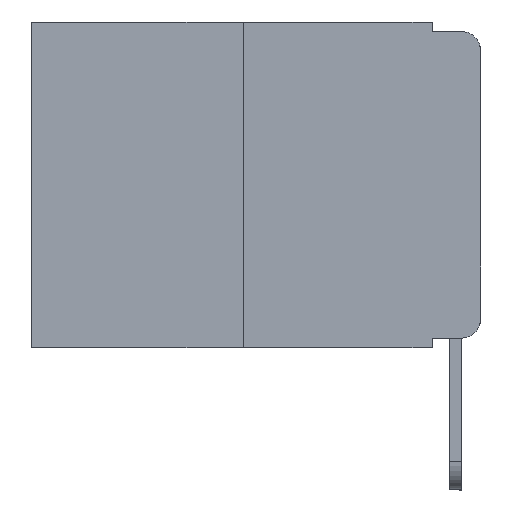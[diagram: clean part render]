
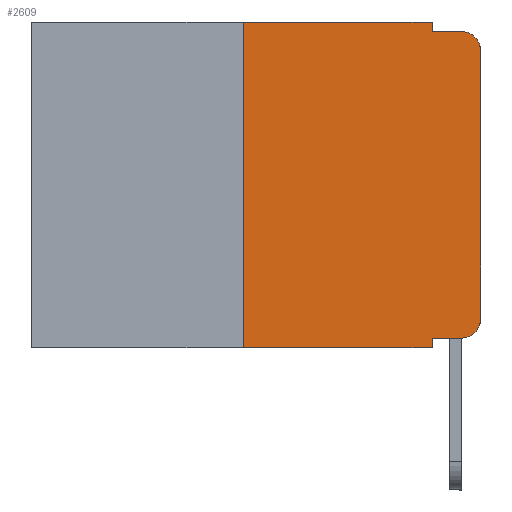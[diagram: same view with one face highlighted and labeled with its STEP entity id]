
A CAD part, left-side view. The second image highlights one B-rep face of the part: STEP entity #2609.
In plain terms, the highlighted planar face has unit normal (-1, 0, 0).
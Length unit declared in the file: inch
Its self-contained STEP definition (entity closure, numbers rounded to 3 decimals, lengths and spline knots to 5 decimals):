
#767 = DIRECTION ( 'NONE',  ( 0., 0., 1. ) ) ;
#901 = AXIS2_PLACEMENT_3D ( 'NONE', #13394, #9608, #2541 ) ;
#1169 = LINE ( 'NONE', #12186, #2252 ) ;
#1453 = VERTEX_POINT ( 'NONE', #3681 ) ;
#1480 = VECTOR ( 'NONE', #8180, 39.37008 ) ;
#2252 = VECTOR ( 'NONE', #17373, 39.37008 ) ;
#2254 = CARTESIAN_POINT ( 'NONE',  ( 0., 0.25, 0. ) ) ;
#2541 = DIRECTION ( 'NONE',  ( 0., 0., -1. ) ) ;
#2609 = ADVANCED_FACE ( 'NONE', ( #9965 ), #8633, .F. ) ;
#2636 = CARTESIAN_POINT ( 'NONE',  ( 0., 0.473, -0.343 ) ) ;
#3166 = EDGE_CURVE ( 'NONE', #3758, #8731, #11826, .T. ) ;
#3441 = EDGE_LOOP ( 'NONE', ( #13390, #12793, #8458, #8248, #9244, #13747, #9294, #8900, #12573, #4435 ) ) ;
#3514 = LINE ( 'NONE', #11663, #14878 ) ;
#3665 = EDGE_CURVE ( 'NONE', #16578, #8731, #12318, .T. ) ;
#3681 = CARTESIAN_POINT ( 'NONE',  ( 0., 0., -0.313 ) ) ;
#3758 = VERTEX_POINT ( 'NONE', #12150 ) ;
#3892 = CARTESIAN_POINT ( 'NONE',  ( 0., 0.051, -0.333 ) ) ;
#4093 = VERTEX_POINT ( 'NONE', #13657 ) ;
#4435 = ORIENTED_EDGE ( 'NONE', *, *, #17539, .T. ) ;
#4487 = DIRECTION ( 'NONE',  ( 0., -1., 0. ) ) ;
#4584 = VECTOR ( 'NONE', #4487, 39.37008 ) ;
#4622 = CARTESIAN_POINT ( 'NONE',  ( 0., 0., 0. ) ) ;
#4822 = CARTESIAN_POINT ( 'NONE',  ( 0., 0.02, -0.01 ) ) ;
#5192 = CARTESIAN_POINT ( 'NONE',  ( 0., 0.02, -0.03 ) ) ;
#5242 = VERTEX_POINT ( 'NONE', #5720 ) ;
#5525 = DIRECTION ( 'NONE',  ( 1., 0., 0. ) ) ;
#5674 = VERTEX_POINT ( 'NONE', #3892 ) ;
#5720 = CARTESIAN_POINT ( 'NONE',  ( 0., 0.02, -0.333 ) ) ;
#5815 = EDGE_CURVE ( 'NONE', #1453, #3758, #6295, .T. ) ;
#6295 = LINE ( 'NONE', #4622, #10656 ) ;
#7098 = LINE ( 'NONE', #8301, #13441 ) ;
#7421 = DIRECTION ( 'NONE',  ( 0., 0., 1. ) ) ;
#8180 = DIRECTION ( 'NONE',  ( 0., -1., 0. ) ) ;
#8186 = DIRECTION ( 'NONE',  ( 0., -1., 0. ) ) ;
#8248 = ORIENTED_EDGE ( 'NONE', *, *, #11457, .F. ) ;
#8301 = CARTESIAN_POINT ( 'NONE',  ( 0., 0.051, 0. ) ) ;
#8458 = ORIENTED_EDGE ( 'NONE', *, *, #3665, .F. ) ;
#8633 = PLANE ( 'NONE',  #9193 ) ;
#8731 = VERTEX_POINT ( 'NONE', #4822 ) ;
#8786 = DIRECTION ( 'NONE',  ( -1., 0., 0. ) ) ;
#8900 = ORIENTED_EDGE ( 'NONE', *, *, #15460, .F. ) ;
#8952 = AXIS2_PLACEMENT_3D ( 'NONE', #5192, #8786, #13424 ) ;
#8954 = VECTOR ( 'NONE', #767, 39.37008 ) ;
#8999 = CARTESIAN_POINT ( 'NONE',  ( 0., 0.25, 0. ) ) ;
#9193 = AXIS2_PLACEMENT_3D ( 'NONE', #14134, #5525, #16583 ) ;
#9244 = ORIENTED_EDGE ( 'NONE', *, *, #15799, .F. ) ;
#9294 = ORIENTED_EDGE ( 'NONE', *, *, #17681, .T. ) ;
#9521 = LINE ( 'NONE', #2636, #1480 ) ;
#9608 = DIRECTION ( 'NONE',  ( -1., 0., 0. ) ) ;
#9965 = FACE_OUTER_BOUND ( 'NONE', #3441, .T. ) ;
#10115 = VERTEX_POINT ( 'NONE', #16074 ) ;
#10433 = LINE ( 'NONE', #8999, #8954 ) ;
#10656 = VECTOR ( 'NONE', #7421, 39.37008 ) ;
#10741 = EDGE_CURVE ( 'NONE', #5674, #5242, #3514, .T. ) ;
#10966 = CARTESIAN_POINT ( 'NONE',  ( 0., 0.051, -0.01 ) ) ;
#11457 = EDGE_CURVE ( 'NONE', #10115, #16578, #7098, .T. ) ;
#11663 = CARTESIAN_POINT ( 'NONE',  ( 0., 0.051, -0.333 ) ) ;
#11826 = CIRCLE ( 'NONE', #8952, 0.02 ) ;
#12150 = CARTESIAN_POINT ( 'NONE',  ( 0., 0., -0.03 ) ) ;
#12186 = CARTESIAN_POINT ( 'NONE',  ( 0., 0.051, 0. ) ) ;
#12318 = LINE ( 'NONE', #10966, #14406 ) ;
#12423 = CIRCLE ( 'NONE', #901, 0.02 ) ;
#12436 = DIRECTION ( 'NONE',  ( 0., 0., -1. ) ) ;
#12573 = ORIENTED_EDGE ( 'NONE', *, *, #10741, .T. ) ;
#12793 = ORIENTED_EDGE ( 'NONE', *, *, #3166, .T. ) ;
#13343 = VERTEX_POINT ( 'NONE', #14663 ) ;
#13390 = ORIENTED_EDGE ( 'NONE', *, *, #5815, .T. ) ;
#13394 = CARTESIAN_POINT ( 'NONE',  ( 0., 0.02, -0.313 ) ) ;
#13424 = DIRECTION ( 'NONE',  ( 0., 0., -1. ) ) ;
#13441 = VECTOR ( 'NONE', #12436, 39.37008 ) ;
#13657 = CARTESIAN_POINT ( 'NONE',  ( 0., 0.25, -0.343 ) ) ;
#13747 = ORIENTED_EDGE ( 'NONE', *, *, #16263, .F. ) ;
#14134 = CARTESIAN_POINT ( 'NONE',  ( 0., 0.473, 0. ) ) ;
#14406 = VECTOR ( 'NONE', #8186, 39.37008 ) ;
#14663 = CARTESIAN_POINT ( 'NONE',  ( 0., 0.051, -0.343 ) ) ;
#14878 = VECTOR ( 'NONE', #15934, 39.37008 ) ;
#15447 = LINE ( 'NONE', #16897, #4584 ) ;
#15460 = EDGE_CURVE ( 'NONE', #5674, #13343, #1169, .T. ) ;
#15762 = CARTESIAN_POINT ( 'NONE',  ( 0., 0.051, -0.01 ) ) ;
#15799 = EDGE_CURVE ( 'NONE', #16724, #10115, #15447, .T. ) ;
#15934 = DIRECTION ( 'NONE',  ( 0., -1., 0. ) ) ;
#16074 = CARTESIAN_POINT ( 'NONE',  ( 0., 0.051, 0. ) ) ;
#16263 = EDGE_CURVE ( 'NONE', #4093, #16724, #10433, .T. ) ;
#16578 = VERTEX_POINT ( 'NONE', #15762 ) ;
#16583 = DIRECTION ( 'NONE',  ( 0., 0., -1. ) ) ;
#16724 = VERTEX_POINT ( 'NONE', #2254 ) ;
#16897 = CARTESIAN_POINT ( 'NONE',  ( 0., 0.473, 0. ) ) ;
#17373 = DIRECTION ( 'NONE',  ( 0., 0., -1. ) ) ;
#17539 = EDGE_CURVE ( 'NONE', #5242, #1453, #12423, .T. ) ;
#17681 = EDGE_CURVE ( 'NONE', #4093, #13343, #9521, .T. ) ;
